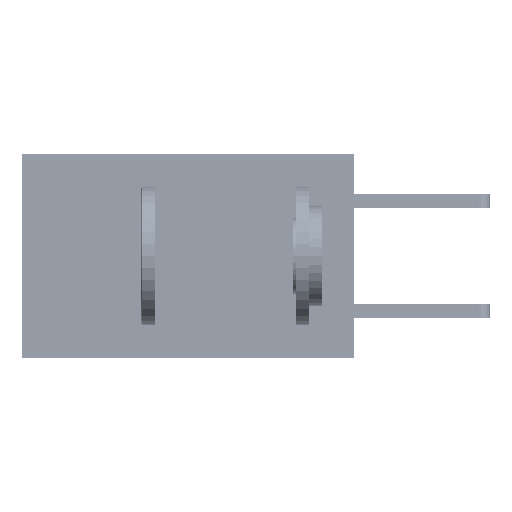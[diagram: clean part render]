
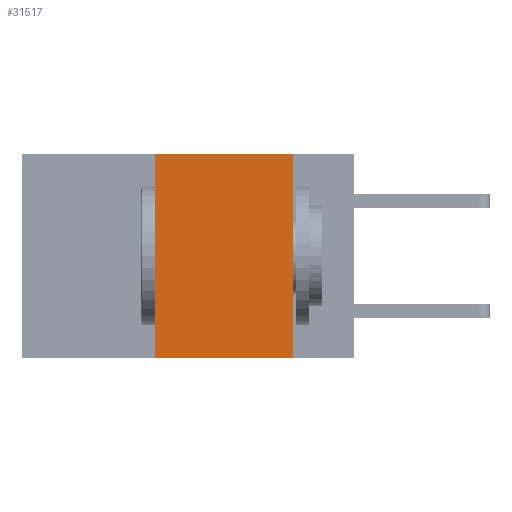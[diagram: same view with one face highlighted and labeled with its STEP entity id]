
A CAD part, left-side view. The second image highlights one B-rep face of the part: STEP entity #31517.
In plain terms, the highlighted planar face has unit normal (-1, 0, 0).
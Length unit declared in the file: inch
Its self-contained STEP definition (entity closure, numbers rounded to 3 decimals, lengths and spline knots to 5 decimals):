
#543 = EDGE_CURVE ( 'NONE', #24968, #13037, #36835, .T. ) ;
#731 = LINE ( 'NONE', #37269, #39930 ) ;
#1632 = ORIENTED_EDGE ( 'NONE', *, *, #31620, .F. ) ;
#2835 = EDGE_CURVE ( 'NONE', #24968, #5697, #42408, .T. ) ;
#2900 = VECTOR ( 'NONE', #15986, 39.37008 ) ;
#3526 = ORIENTED_EDGE ( 'NONE', *, *, #543, .F. ) ;
#5365 = CARTESIAN_POINT ( 'NONE',  ( 0., 0.11, -0.37 ) ) ;
#5697 = VERTEX_POINT ( 'NONE', #5365 ) ;
#6303 = CARTESIAN_POINT ( 'NONE',  ( 0., 0.36, 0. ) ) ;
#6591 = ORIENTED_EDGE ( 'NONE', *, *, #10029, .F. ) ;
#8190 = CARTESIAN_POINT ( 'NONE',  ( 0., 0.36, -0.37 ) ) ;
#10029 = EDGE_CURVE ( 'NONE', #37571, #5697, #731, .T. ) ;
#10176 = FACE_OUTER_BOUND ( 'NONE', #38927, .T. ) ;
#10531 = DIRECTION ( 'NONE',  ( 0., 0., -1. ) ) ;
#11040 = CARTESIAN_POINT ( 'NONE',  ( 0., 0.6, -0.37 ) ) ;
#12164 = CARTESIAN_POINT ( 'NONE',  ( 0., 0.36, 0. ) ) ;
#13037 = VERTEX_POINT ( 'NONE', #6303 ) ;
#15479 = DIRECTION ( 'NONE',  ( 0., 0., -1. ) ) ;
#15986 = DIRECTION ( 'NONE',  ( 0., -1., 0. ) ) ;
#17772 = CARTESIAN_POINT ( 'NONE',  ( 0., 0.11, 0. ) ) ;
#24968 = VERTEX_POINT ( 'NONE', #8190 ) ;
#26209 = DIRECTION ( 'NONE',  ( 0., -1., 0. ) ) ;
#26792 = VECTOR ( 'NONE', #26209, 39.37008 ) ;
#28056 = AXIS2_PLACEMENT_3D ( 'NONE', #34665, #38680, #15479 ) ;
#31517 = ADVANCED_FACE ( 'NONE', ( #10176 ), #46288, .F. ) ;
#31620 = EDGE_CURVE ( 'NONE', #13037, #37571, #46904, .T. ) ;
#33232 = VECTOR ( 'NONE', #35362, 39.37008 ) ;
#34665 = CARTESIAN_POINT ( 'NONE',  ( 0., 0.6, 0. ) ) ;
#35362 = DIRECTION ( 'NONE',  ( 0., 0., 1. ) ) ;
#36835 = LINE ( 'NONE', #12164, #33232 ) ;
#37269 = CARTESIAN_POINT ( 'NONE',  ( 0., 0.11, 0. ) ) ;
#37571 = VERTEX_POINT ( 'NONE', #17772 ) ;
#38680 = DIRECTION ( 'NONE',  ( 1., 0., 0. ) ) ;
#38927 = EDGE_LOOP ( 'NONE', ( #6591, #1632, #3526, #44345 ) ) ;
#39930 = VECTOR ( 'NONE', #10531, 39.37008 ) ;
#42408 = LINE ( 'NONE', #11040, #26792 ) ;
#42704 = CARTESIAN_POINT ( 'NONE',  ( 0., 0.6, 0. ) ) ;
#44345 = ORIENTED_EDGE ( 'NONE', *, *, #2835, .T. ) ;
#46288 = PLANE ( 'NONE',  #28056 ) ;
#46904 = LINE ( 'NONE', #42704, #2900 ) ;
